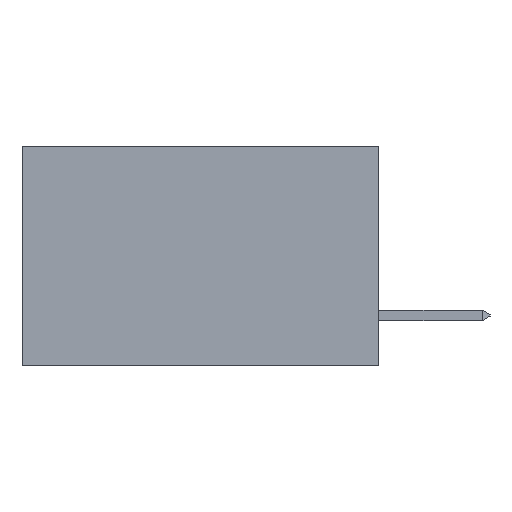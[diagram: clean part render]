
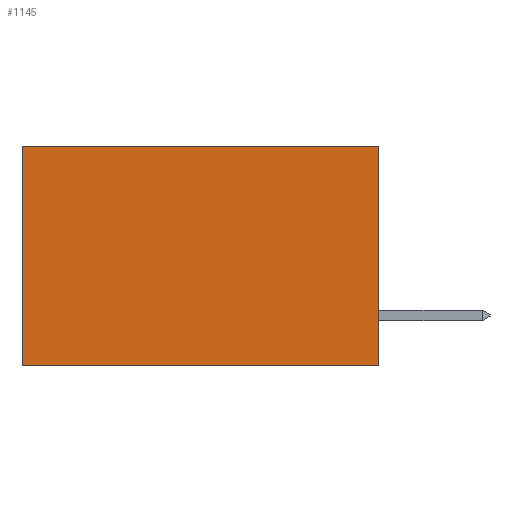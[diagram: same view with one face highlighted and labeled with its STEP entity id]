
A CAD part, left-side view. The second image highlights one B-rep face of the part: STEP entity #1145.
In plain terms, the highlighted planar face has unit normal (-1, 0, 0).
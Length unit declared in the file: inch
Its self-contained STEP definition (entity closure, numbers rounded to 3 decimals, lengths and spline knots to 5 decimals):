
#300 = EDGE_CURVE ( 'NONE', #9062, #3165, #3271, .T. ) ;
#676 = CARTESIAN_POINT ( 'NONE',  ( 0.2615, 0., -0.37 ) ) ;
#767 = CARTESIAN_POINT ( 'NONE',  ( 0.2615, 0., -0.37 ) ) ;
#844 = EDGE_CURVE ( 'NONE', #3165, #9969, #1958, .T. ) ;
#1127 = VECTOR ( 'NONE', #11018, 39.37008 ) ;
#1145 = ADVANCED_FACE ( 'NONE', ( #7726 ), #8973, .F. ) ;
#1750 = LINE ( 'NONE', #10462, #3816 ) ;
#1958 = LINE ( 'NONE', #10081, #10571 ) ;
#2038 = ORIENTED_EDGE ( 'NONE', *, *, #6588, .F. ) ;
#2193 = VECTOR ( 'NONE', #9158, 39.37008 ) ;
#2334 = ORIENTED_EDGE ( 'NONE', *, *, #300, .T. ) ;
#3165 = VERTEX_POINT ( 'NONE', #10624 ) ;
#3222 = CARTESIAN_POINT ( 'NONE',  ( 0.2615, 0., 0. ) ) ;
#3271 = LINE ( 'NONE', #5720, #1127 ) ;
#3816 = VECTOR ( 'NONE', #9306, 39.37008 ) ;
#4457 = AXIS2_PLACEMENT_3D ( 'NONE', #5979, #8526, #6218 ) ;
#5720 = CARTESIAN_POINT ( 'NONE',  ( 0.2615, 0., 0. ) ) ;
#5979 = CARTESIAN_POINT ( 'NONE',  ( 0.2615, 0., -0.37 ) ) ;
#6203 = VERTEX_POINT ( 'NONE', #767 ) ;
#6218 = DIRECTION ( 'NONE',  ( 0., 0., -1. ) ) ;
#6478 = DIRECTION ( 'NONE',  ( 0., 0., -1. ) ) ;
#6588 = EDGE_CURVE ( 'NONE', #9062, #6203, #9101, .T. ) ;
#7263 = EDGE_CURVE ( 'NONE', #6203, #9969, #1750, .T. ) ;
#7307 = EDGE_LOOP ( 'NONE', ( #8441, #10639, #2038, #2334 ) ) ;
#7726 = FACE_OUTER_BOUND ( 'NONE', #7307, .T. ) ;
#8441 = ORIENTED_EDGE ( 'NONE', *, *, #844, .T. ) ;
#8526 = DIRECTION ( 'NONE',  ( 1., 0., 0. ) ) ;
#8973 = PLANE ( 'NONE',  #4457 ) ;
#9062 = VERTEX_POINT ( 'NONE', #3222 ) ;
#9101 = LINE ( 'NONE', #676, #2193 ) ;
#9158 = DIRECTION ( 'NONE',  ( 0., 0., -1. ) ) ;
#9306 = DIRECTION ( 'NONE',  ( 0., 1., 0. ) ) ;
#9969 = VERTEX_POINT ( 'NONE', #10327 ) ;
#10081 = CARTESIAN_POINT ( 'NONE',  ( 0.2615, 0.6, -0.37 ) ) ;
#10327 = CARTESIAN_POINT ( 'NONE',  ( 0.2615, 0.6, -0.37 ) ) ;
#10462 = CARTESIAN_POINT ( 'NONE',  ( 0.2615, 0., -0.37 ) ) ;
#10571 = VECTOR ( 'NONE', #6478, 39.37008 ) ;
#10624 = CARTESIAN_POINT ( 'NONE',  ( 0.2615, 0.6, 0. ) ) ;
#10639 = ORIENTED_EDGE ( 'NONE', *, *, #7263, .F. ) ;
#11018 = DIRECTION ( 'NONE',  ( 0., 1., 0. ) ) ;
